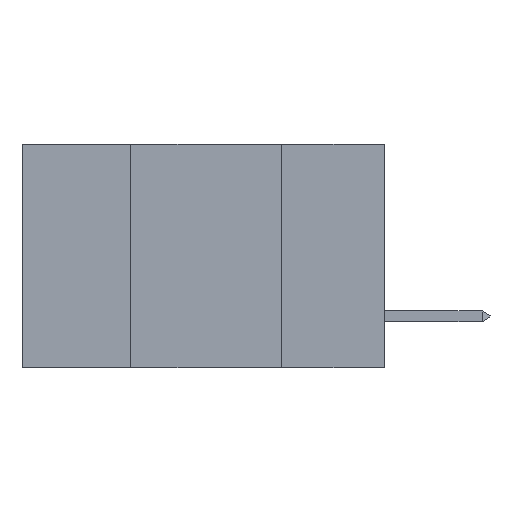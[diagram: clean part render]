
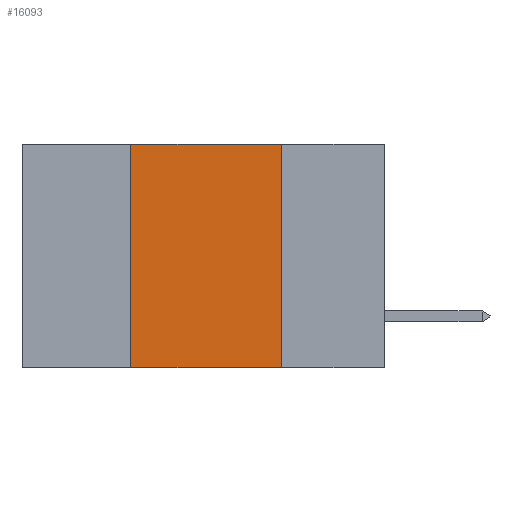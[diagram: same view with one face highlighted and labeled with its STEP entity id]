
A CAD part, left-side view. The second image highlights one B-rep face of the part: STEP entity #16093.
In plain terms, the highlighted planar face has unit normal (-1, 0, 0).
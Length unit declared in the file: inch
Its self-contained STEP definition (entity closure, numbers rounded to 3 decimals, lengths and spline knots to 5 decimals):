
#817 = CARTESIAN_POINT ( 'NONE',  ( 0., 0.6, 0. ) ) ;
#1295 = DIRECTION ( 'NONE',  ( 0., -1., 0. ) ) ;
#1591 = CARTESIAN_POINT ( 'NONE',  ( 0., 0.42, 0. ) ) ;
#2239 = LINE ( 'NONE', #9542, #15031 ) ;
#2333 = EDGE_CURVE ( 'NONE', #7914, #11938, #5200, .T. ) ;
#2556 = CARTESIAN_POINT ( 'NONE',  ( 0., 0.6, 0. ) ) ;
#3065 = VERTEX_POINT ( 'NONE', #10466 ) ;
#4670 = DIRECTION ( 'NONE',  ( 0., -1., 0. ) ) ;
#4708 = VECTOR ( 'NONE', #5596, 39.37008 ) ;
#5101 = DIRECTION ( 'NONE',  ( 0., 0., -1. ) ) ;
#5162 = CARTESIAN_POINT ( 'NONE',  ( 0., 0.42, 0. ) ) ;
#5200 = LINE ( 'NONE', #2556, #17199 ) ;
#5578 = EDGE_CURVE ( 'NONE', #3065, #10951, #10179, .T. ) ;
#5596 = DIRECTION ( 'NONE',  ( 0., 0., 1. ) ) ;
#5921 = EDGE_LOOP ( 'NONE', ( #7117, #6415, #12524, #11030 ) ) ;
#6415 = ORIENTED_EDGE ( 'NONE', *, *, #2333, .F. ) ;
#6496 = FACE_OUTER_BOUND ( 'NONE', #5921, .T. ) ;
#6845 = AXIS2_PLACEMENT_3D ( 'NONE', #817, #13458, #5101 ) ;
#7117 = ORIENTED_EDGE ( 'NONE', *, *, #7188, .F. ) ;
#7188 = EDGE_CURVE ( 'NONE', #11938, #10951, #2239, .T. ) ;
#7879 = PLANE ( 'NONE',  #6845 ) ;
#7914 = VERTEX_POINT ( 'NONE', #5162 ) ;
#9542 = CARTESIAN_POINT ( 'NONE',  ( 0., 0.17, 0. ) ) ;
#9707 = VECTOR ( 'NONE', #4670, 39.37008 ) ;
#10179 = LINE ( 'NONE', #12855, #9707 ) ;
#10466 = CARTESIAN_POINT ( 'NONE',  ( 0., 0.42, -0.37 ) ) ;
#10951 = VERTEX_POINT ( 'NONE', #14229 ) ;
#11030 = ORIENTED_EDGE ( 'NONE', *, *, #5578, .T. ) ;
#11938 = VERTEX_POINT ( 'NONE', #13231 ) ;
#12524 = ORIENTED_EDGE ( 'NONE', *, *, #14100, .F. ) ;
#12855 = CARTESIAN_POINT ( 'NONE',  ( 0., 0.6, -0.37 ) ) ;
#13231 = CARTESIAN_POINT ( 'NONE',  ( 0., 0.17, 0. ) ) ;
#13413 = DIRECTION ( 'NONE',  ( 0., 0., -1. ) ) ;
#13458 = DIRECTION ( 'NONE',  ( 1., 0., 0. ) ) ;
#14100 = EDGE_CURVE ( 'NONE', #3065, #7914, #16862, .T. ) ;
#14229 = CARTESIAN_POINT ( 'NONE',  ( 0., 0.17, -0.37 ) ) ;
#15031 = VECTOR ( 'NONE', #13413, 39.37008 ) ;
#16093 = ADVANCED_FACE ( 'NONE', ( #6496 ), #7879, .F. ) ;
#16862 = LINE ( 'NONE', #1591, #4708 ) ;
#17199 = VECTOR ( 'NONE', #1295, 39.37008 ) ;
